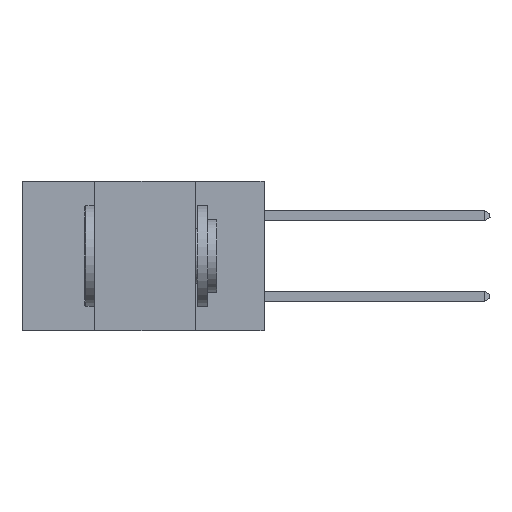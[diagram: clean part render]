
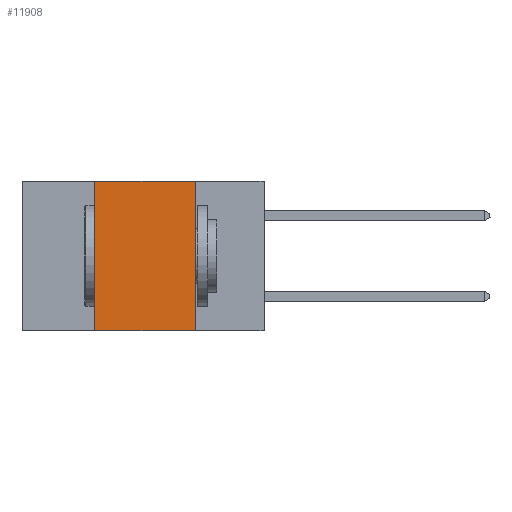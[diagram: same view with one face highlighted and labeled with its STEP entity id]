
A CAD part, left-side view. The second image highlights one B-rep face of the part: STEP entity #11908.
In plain terms, the highlighted planar face has unit normal (-1, 0, 0).
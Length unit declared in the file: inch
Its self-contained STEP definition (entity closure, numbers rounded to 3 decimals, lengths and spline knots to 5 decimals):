
#46 = CARTESIAN_POINT ( 'NONE',  ( 0., 0.6, 0. ) ) ;
#581 = CARTESIAN_POINT ( 'NONE',  ( 0., 0.6, -0.37 ) ) ;
#823 = CARTESIAN_POINT ( 'NONE',  ( 0., 0.17, 0. ) ) ;
#1192 = LINE ( 'NONE', #581, #4106 ) ;
#1983 = AXIS2_PLACEMENT_3D ( 'NONE', #46, #7102, #11293 ) ;
#2272 = DIRECTION ( 'NONE',  ( 0., 0., -1. ) ) ;
#3505 = ORIENTED_EDGE ( 'NONE', *, *, #13161, .F. ) ;
#3559 = DIRECTION ( 'NONE',  ( 0., -1., 0. ) ) ;
#3908 = LINE ( 'NONE', #17948, #15585 ) ;
#4106 = VECTOR ( 'NONE', #17654, 39.37008 ) ;
#4527 = EDGE_CURVE ( 'NONE', #13868, #4965, #8848, .T. ) ;
#4602 = LINE ( 'NONE', #823, #16248 ) ;
#4947 = EDGE_LOOP ( 'NONE', ( #5505, #15704, #3505, #7806 ) ) ;
#4965 = VERTEX_POINT ( 'NONE', #16074 ) ;
#5259 = DIRECTION ( 'NONE',  ( 0., 0., 1. ) ) ;
#5505 = ORIENTED_EDGE ( 'NONE', *, *, #16353, .F. ) ;
#5966 = EDGE_CURVE ( 'NONE', #14110, #8642, #1192, .T. ) ;
#7102 = DIRECTION ( 'NONE',  ( 1., 0., 0. ) ) ;
#7806 = ORIENTED_EDGE ( 'NONE', *, *, #5966, .T. ) ;
#8601 = PLANE ( 'NONE',  #1983 ) ;
#8642 = VERTEX_POINT ( 'NONE', #17143 ) ;
#8848 = LINE ( 'NONE', #16327, #14467 ) ;
#11293 = DIRECTION ( 'NONE',  ( 0., 0., -1. ) ) ;
#11908 = ADVANCED_FACE ( 'NONE', ( #18388 ), #8601, .F. ) ;
#13161 = EDGE_CURVE ( 'NONE', #14110, #13868, #3908, .T. ) ;
#13868 = VERTEX_POINT ( 'NONE', #16939 ) ;
#14110 = VERTEX_POINT ( 'NONE', #16998 ) ;
#14467 = VECTOR ( 'NONE', #3559, 39.37008 ) ;
#15585 = VECTOR ( 'NONE', #5259, 39.37008 ) ;
#15704 = ORIENTED_EDGE ( 'NONE', *, *, #4527, .F. ) ;
#16074 = CARTESIAN_POINT ( 'NONE',  ( 0., 0.17, 0. ) ) ;
#16248 = VECTOR ( 'NONE', #2272, 39.37008 ) ;
#16327 = CARTESIAN_POINT ( 'NONE',  ( 0., 0.6, 0. ) ) ;
#16353 = EDGE_CURVE ( 'NONE', #4965, #8642, #4602, .T. ) ;
#16939 = CARTESIAN_POINT ( 'NONE',  ( 0., 0.42, 0. ) ) ;
#16998 = CARTESIAN_POINT ( 'NONE',  ( 0., 0.42, -0.37 ) ) ;
#17143 = CARTESIAN_POINT ( 'NONE',  ( 0., 0.17, -0.37 ) ) ;
#17654 = DIRECTION ( 'NONE',  ( 0., -1., 0. ) ) ;
#17948 = CARTESIAN_POINT ( 'NONE',  ( 0., 0.42, 0. ) ) ;
#18388 = FACE_OUTER_BOUND ( 'NONE', #4947, .T. ) ;
